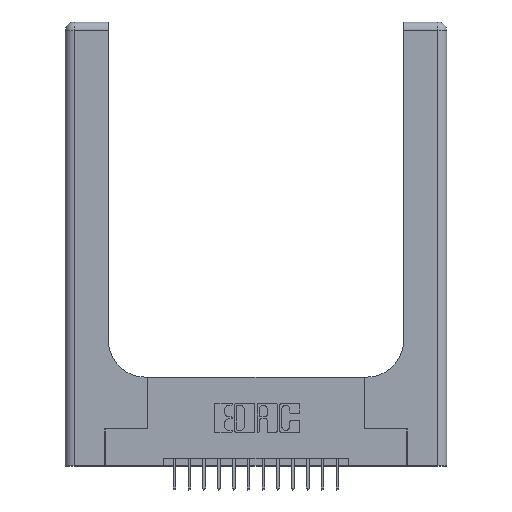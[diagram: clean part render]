
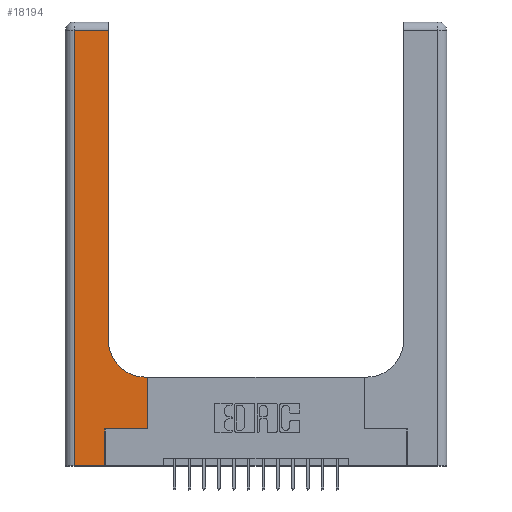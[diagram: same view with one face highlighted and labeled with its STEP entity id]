
A CAD part, top view. The second image highlights one B-rep face of the part: STEP entity #18194.
In plain terms, the highlighted planar face has unit normal (0, 0, 1).
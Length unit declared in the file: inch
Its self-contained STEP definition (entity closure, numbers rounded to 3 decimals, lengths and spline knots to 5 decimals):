
#71 = CARTESIAN_POINT ( 'NONE',  ( 0.06, 0., 0.37 ) ) ;
#383 = LINE ( 'NONE', #6642, #4357 ) ;
#414 = CARTESIAN_POINT ( 'NONE',  ( 0.2915, 2.94, 0.37 ) ) ;
#426 = PLANE ( 'NONE',  #10249 ) ;
#529 = CARTESIAN_POINT ( 'NONE',  ( 0.2915, 0.85, 0.37 ) ) ;
#586 = ORIENTED_EDGE ( 'NONE', *, *, #14330, .T. ) ;
#778 = VECTOR ( 'NONE', #14522, 39.37008 ) ;
#1309 = CARTESIAN_POINT ( 'NONE',  ( 0.269, 0., 0.37 ) ) ;
#1341 = VERTEX_POINT ( 'NONE', #10681 ) ;
#1747 = CARTESIAN_POINT ( 'NONE',  ( 0.5415, 0.85, 0.37 ) ) ;
#2645 = DIRECTION ( 'NONE',  ( -1., 0., 0. ) ) ;
#2851 = DIRECTION ( 'NONE',  ( 0., -1., 0. ) ) ;
#2990 = CARTESIAN_POINT ( 'NONE',  ( 0.2915, 0.6, 0.37 ) ) ;
#3264 = DIRECTION ( 'NONE',  ( 1., 0., 0. ) ) ;
#3454 = DIRECTION ( 'NONE',  ( 0., 0., -1. ) ) ;
#3627 = LINE ( 'NONE', #3960, #13761 ) ;
#3681 = EDGE_CURVE ( 'NONE', #16478, #1341, #11646, .T. ) ;
#3960 = CARTESIAN_POINT ( 'NONE',  ( 0.5585, 0.25, 0.37 ) ) ;
#4020 = VERTEX_POINT ( 'NONE', #414 ) ;
#4092 = CARTESIAN_POINT ( 'NONE',  ( 0.5585, 0.25, 0.37 ) ) ;
#4117 = VECTOR ( 'NONE', #14460, 39.37008 ) ;
#4132 = VECTOR ( 'NONE', #11553, 39.37008 ) ;
#4357 = VECTOR ( 'NONE', #8139, 39.37008 ) ;
#4477 = CARTESIAN_POINT ( 'NONE',  ( 0.269, 0.25, 0.37 ) ) ;
#4508 = FACE_OUTER_BOUND ( 'NONE', #8817, .T. ) ;
#4600 = LINE ( 'NONE', #1309, #4132 ) ;
#4754 = LINE ( 'NONE', #4477, #778 ) ;
#4920 = EDGE_CURVE ( 'NONE', #7460, #7778, #16474, .T. ) ;
#5453 = ORIENTED_EDGE ( 'NONE', *, *, #14549, .T. ) ;
#5840 = CARTESIAN_POINT ( 'NONE',  ( 0.06, 3., 0.37 ) ) ;
#6333 = AXIS2_PLACEMENT_3D ( 'NONE', #1747, #11960, #3264 ) ;
#6361 = LINE ( 'NONE', #15829, #13964 ) ;
#6642 = CARTESIAN_POINT ( 'NONE',  ( 0., 2.94, 0.37 ) ) ;
#7176 = EDGE_CURVE ( 'NONE', #11048, #16478, #3627, .T. ) ;
#7342 = DIRECTION ( 'NONE',  ( 0., 1., 0. ) ) ;
#7446 = ORIENTED_EDGE ( 'NONE', *, *, #15049, .T. ) ;
#7460 = VERTEX_POINT ( 'NONE', #71 ) ;
#7778 = VERTEX_POINT ( 'NONE', #15553 ) ;
#8139 = DIRECTION ( 'NONE',  ( -1., 0., 0. ) ) ;
#8406 = DIRECTION ( 'NONE',  ( 0., 1., 0. ) ) ;
#8711 = LINE ( 'NONE', #5840, #17116 ) ;
#8817 = EDGE_LOOP ( 'NONE', ( #15524, #5453, #7446, #16257, #586, #18571, #16111, #8995, #17389 ) ) ;
#8995 = ORIENTED_EDGE ( 'NONE', *, *, #3681, .T. ) ;
#10249 = AXIS2_PLACEMENT_3D ( 'NONE', #12127, #3454, #13544 ) ;
#10286 = VERTEX_POINT ( 'NONE', #529 ) ;
#10623 = EDGE_CURVE ( 'NONE', #10286, #4020, #6361, .T. ) ;
#10681 = CARTESIAN_POINT ( 'NONE',  ( 0.5415, 0.6, 0.37 ) ) ;
#10772 = EDGE_CURVE ( 'NONE', #1341, #10286, #11754, .T. ) ;
#11048 = VERTEX_POINT ( 'NONE', #4092 ) ;
#11553 = DIRECTION ( 'NONE',  ( 0., 1., 0. ) ) ;
#11646 = LINE ( 'NONE', #2990, #15828 ) ;
#11754 = CIRCLE ( 'NONE', #6333, 0.25 ) ;
#11905 = CARTESIAN_POINT ( 'NONE',  ( 0.5585, 0.6, 0.37 ) ) ;
#11960 = DIRECTION ( 'NONE',  ( 0., 0., -1. ) ) ;
#12127 = CARTESIAN_POINT ( 'NONE',  ( 0., 3., 0.37 ) ) ;
#13359 = CARTESIAN_POINT ( 'NONE',  ( 0.269, 0.25, 0.37 ) ) ;
#13544 = DIRECTION ( 'NONE',  ( -1., 0., 0. ) ) ;
#13761 = VECTOR ( 'NONE', #8406, 39.37008 ) ;
#13924 = VERTEX_POINT ( 'NONE', #13359 ) ;
#13964 = VECTOR ( 'NONE', #7342, 39.37008 ) ;
#14330 = EDGE_CURVE ( 'NONE', #7778, #13924, #4600, .T. ) ;
#14460 = DIRECTION ( 'NONE',  ( 1., 0., 0. ) ) ;
#14522 = DIRECTION ( 'NONE',  ( 1., 0., 0. ) ) ;
#14549 = EDGE_CURVE ( 'NONE', #4020, #15345, #383, .T. ) ;
#15049 = EDGE_CURVE ( 'NONE', #15345, #7460, #8711, .T. ) ;
#15345 = VERTEX_POINT ( 'NONE', #16509 ) ;
#15524 = ORIENTED_EDGE ( 'NONE', *, *, #10623, .T. ) ;
#15553 = CARTESIAN_POINT ( 'NONE',  ( 0.269, 0., 0.37 ) ) ;
#15828 = VECTOR ( 'NONE', #2645, 39.37008 ) ;
#15829 = CARTESIAN_POINT ( 'NONE',  ( 0.2915, 3., 0.37 ) ) ;
#16111 = ORIENTED_EDGE ( 'NONE', *, *, #7176, .T. ) ;
#16257 = ORIENTED_EDGE ( 'NONE', *, *, #4920, .T. ) ;
#16474 = LINE ( 'NONE', #18655, #4117 ) ;
#16478 = VERTEX_POINT ( 'NONE', #11905 ) ;
#16509 = CARTESIAN_POINT ( 'NONE',  ( 0.06, 2.94, 0.37 ) ) ;
#17116 = VECTOR ( 'NONE', #2851, 39.37008 ) ;
#17389 = ORIENTED_EDGE ( 'NONE', *, *, #10772, .T. ) ;
#18000 = EDGE_CURVE ( 'NONE', #13924, #11048, #4754, .T. ) ;
#18194 = ADVANCED_FACE ( 'NONE', ( #4508 ), #426, .F. ) ;
#18571 = ORIENTED_EDGE ( 'NONE', *, *, #18000, .T. ) ;
#18655 = CARTESIAN_POINT ( 'NONE',  ( 0., 0., 0.37 ) ) ;
